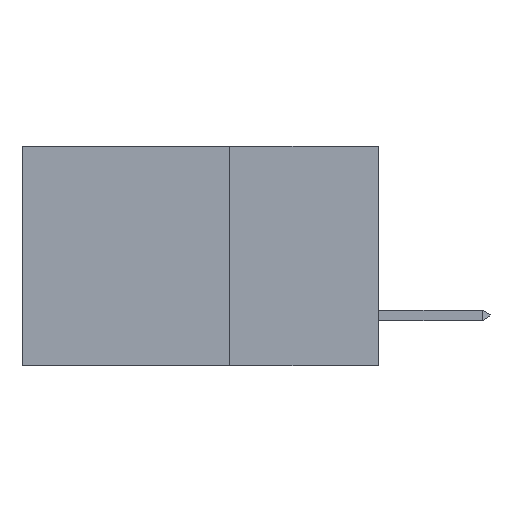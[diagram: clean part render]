
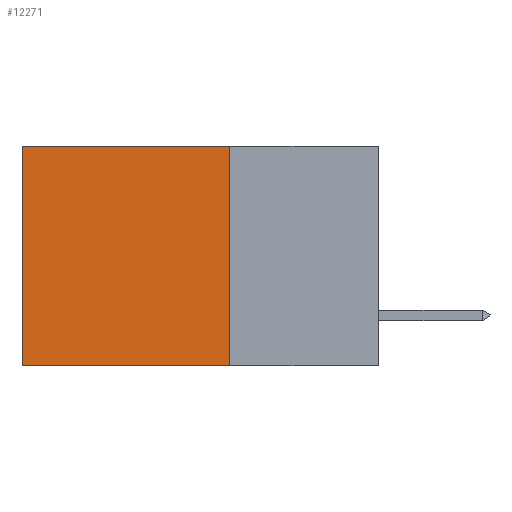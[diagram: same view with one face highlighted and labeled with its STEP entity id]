
A CAD part, left-side view. The second image highlights one B-rep face of the part: STEP entity #12271.
In plain terms, the highlighted planar face has unit normal (-1, 0, 0).
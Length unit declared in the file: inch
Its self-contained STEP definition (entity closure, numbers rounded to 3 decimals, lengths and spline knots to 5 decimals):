
#517 = CARTESIAN_POINT ( 'NONE',  ( 0.2615, 0.6, -0.37 ) ) ;
#850 = DIRECTION ( 'NONE',  ( 0., 1., 0. ) ) ;
#928 = EDGE_CURVE ( 'NONE', #9547, #8147, #17941, .T. ) ;
#1103 = LINE ( 'NONE', #1204, #11299 ) ;
#1204 = CARTESIAN_POINT ( 'NONE',  ( 0.2615, 0.25, 0. ) ) ;
#1954 = FACE_OUTER_BOUND ( 'NONE', #12053, .T. ) ;
#2149 = DIRECTION ( 'NONE',  ( 1., 0., 0. ) ) ;
#2252 = CARTESIAN_POINT ( 'NONE',  ( 0.2615, 0.25, -0.37 ) ) ;
#3541 = DIRECTION ( 'NONE',  ( 0., 0., -1. ) ) ;
#3732 = CARTESIAN_POINT ( 'NONE',  ( 0.2615, 0.25, -0.37 ) ) ;
#3761 = CARTESIAN_POINT ( 'NONE',  ( 0.2615, 0.25, 0. ) ) ;
#4554 = ORIENTED_EDGE ( 'NONE', *, *, #9614, .T. ) ;
#6584 = DIRECTION ( 'NONE',  ( 0., 0., -1. ) ) ;
#7938 = AXIS2_PLACEMENT_3D ( 'NONE', #13993, #2149, #3541 ) ;
#7989 = PLANE ( 'NONE',  #7938 ) ;
#8147 = VERTEX_POINT ( 'NONE', #517 ) ;
#8398 = VECTOR ( 'NONE', #18135, 39.37008 ) ;
#9547 = VERTEX_POINT ( 'NONE', #12667 ) ;
#9614 = EDGE_CURVE ( 'NONE', #11883, #9547, #1103, .T. ) ;
#11299 = VECTOR ( 'NONE', #14527, 39.37008 ) ;
#11883 = VERTEX_POINT ( 'NONE', #3761 ) ;
#12053 = EDGE_LOOP ( 'NONE', ( #17993, #15462, #13185, #4554 ) ) ;
#12271 = ADVANCED_FACE ( 'NONE', ( #1954 ), #7989, .F. ) ;
#12302 = EDGE_CURVE ( 'NONE', #14930, #8147, #15774, .T. ) ;
#12667 = CARTESIAN_POINT ( 'NONE',  ( 0.2615, 0.6, 0. ) ) ;
#13185 = ORIENTED_EDGE ( 'NONE', *, *, #16512, .F. ) ;
#13993 = CARTESIAN_POINT ( 'NONE',  ( 0.2615, 0.25, -0.37 ) ) ;
#14527 = DIRECTION ( 'NONE',  ( 0., 1., 0. ) ) ;
#14930 = VERTEX_POINT ( 'NONE', #16447 ) ;
#15253 = CARTESIAN_POINT ( 'NONE',  ( 0.2615, 0.6, -0.37 ) ) ;
#15462 = ORIENTED_EDGE ( 'NONE', *, *, #12302, .F. ) ;
#15464 = LINE ( 'NONE', #3732, #16832 ) ;
#15774 = LINE ( 'NONE', #2252, #18961 ) ;
#16447 = CARTESIAN_POINT ( 'NONE',  ( 0.2615, 0.25, -0.37 ) ) ;
#16512 = EDGE_CURVE ( 'NONE', #11883, #14930, #15464, .T. ) ;
#16832 = VECTOR ( 'NONE', #6584, 39.37008 ) ;
#17941 = LINE ( 'NONE', #15253, #8398 ) ;
#17993 = ORIENTED_EDGE ( 'NONE', *, *, #928, .T. ) ;
#18135 = DIRECTION ( 'NONE',  ( 0., 0., -1. ) ) ;
#18961 = VECTOR ( 'NONE', #850, 39.37008 ) ;
